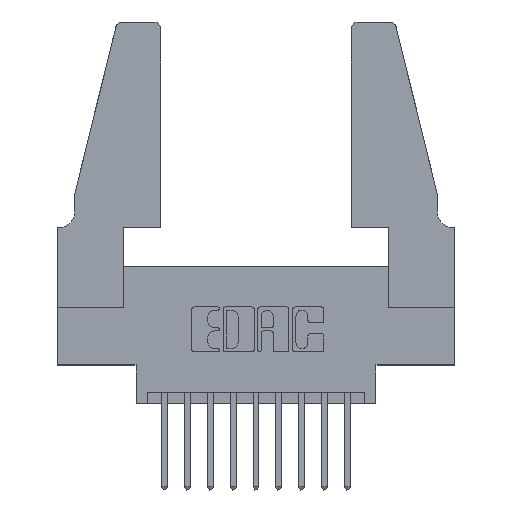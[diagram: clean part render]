
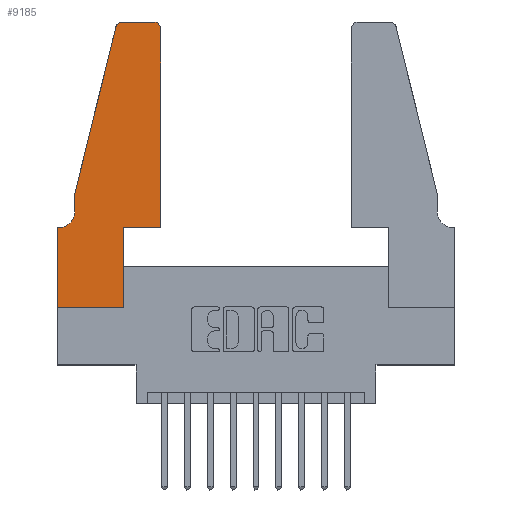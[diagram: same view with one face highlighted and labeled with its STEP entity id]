
A CAD part, top view. The second image highlights one B-rep face of the part: STEP entity #9185.
In plain terms, the highlighted planar face has unit normal (0, 0, 1).
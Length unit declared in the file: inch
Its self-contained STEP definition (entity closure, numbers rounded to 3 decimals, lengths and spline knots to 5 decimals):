
#111 = ORIENTED_EDGE ( 'NONE', *, *, #8602, .T. ) ;
#205 = FACE_OUTER_BOUND ( 'NONE', #3794, .T. ) ;
#253 = AXIS2_PLACEMENT_3D ( 'NONE', #5200, #1895, #12442 ) ;
#400 = EDGE_CURVE ( 'NONE', #8522, #9826, #4675, .T. ) ;
#411 = ORIENTED_EDGE ( 'NONE', *, *, #6340, .T. ) ;
#1037 = AXIS2_PLACEMENT_3D ( 'NONE', #12766, #9721, #3283 ) ;
#1057 = CARTESIAN_POINT ( 'NONE',  ( 0.284, 1.22, 0.37 ) ) ;
#1228 = CARTESIAN_POINT ( 'NONE',  ( 0., 0.35, 0.37 ) ) ;
#1343 = EDGE_CURVE ( 'NONE', #1656, #9816, #12976, .T. ) ;
#1396 = CARTESIAN_POINT ( 'NONE',  ( 0.2865, 0., 0.37 ) ) ;
#1656 = VERTEX_POINT ( 'NONE', #8082 ) ;
#1895 = DIRECTION ( 'NONE',  ( 0., 0., -1. ) ) ;
#2164 = ORIENTED_EDGE ( 'NONE', *, *, #400, .T. ) ;
#2370 = DIRECTION ( 'NONE',  ( -1., 0., 0. ) ) ;
#2409 = CARTESIAN_POINT ( 'NONE',  ( 0.4205, 1.25, 0.37 ) ) ;
#2418 = LINE ( 'NONE', #12150, #4247 ) ;
#2682 = CARTESIAN_POINT ( 'NONE',  ( 0.4505, 0.35, 0.37 ) ) ;
#2953 = CIRCLE ( 'NONE', #13236, 0.03 ) ;
#3154 = VERTEX_POINT ( 'NONE', #13482 ) ;
#3175 = CARTESIAN_POINT ( 'NONE',  ( 0.0755, 0.35, 0.37 ) ) ;
#3195 = LINE ( 'NONE', #11747, #11342 ) ;
#3283 = DIRECTION ( 'NONE',  ( 1., 0., 0. ) ) ;
#3365 = DIRECTION ( 'NONE',  ( 1., 0., 0. ) ) ;
#3552 = DIRECTION ( 'NONE',  ( 0., 0., 1. ) ) ;
#3661 = CARTESIAN_POINT ( 'NONE',  ( 0.4505, 1.22, 0.37 ) ) ;
#3710 = EDGE_CURVE ( 'NONE', #9374, #10309, #12224, .T. ) ;
#3794 = EDGE_LOOP ( 'NONE', ( #12296, #4757, #111, #2164, #6832, #6140, #9822, #10789, #10201, #5926, #411, #8245 ) ) ;
#4059 = DIRECTION ( 'NONE',  ( 0., 0., 1. ) ) ;
#4098 = CARTESIAN_POINT ( 'NONE',  ( 0.2865, 0.35, 0.37 ) ) ;
#4234 = DIRECTION ( 'NONE',  ( 0., 1., 0. ) ) ;
#4247 = VECTOR ( 'NONE', #11292, 39.37008 ) ;
#4675 = LINE ( 'NONE', #10441, #12673 ) ;
#4757 = ORIENTED_EDGE ( 'NONE', *, *, #11377, .T. ) ;
#4769 = CARTESIAN_POINT ( 'NONE',  ( 0., 0., 0.37 ) ) ;
#5063 = CARTESIAN_POINT ( 'NONE',  ( 0.284, 1.25, 0.37 ) ) ;
#5200 = CARTESIAN_POINT ( 'NONE',  ( 0.0055, 0.42, 0.37 ) ) ;
#5499 = VERTEX_POINT ( 'NONE', #10405 ) ;
#5926 = ORIENTED_EDGE ( 'NONE', *, *, #8165, .T. ) ;
#6053 = VECTOR ( 'NONE', #13142, 39.37008 ) ;
#6140 = ORIENTED_EDGE ( 'NONE', *, *, #1343, .T. ) ;
#6340 = EDGE_CURVE ( 'NONE', #3154, #7685, #3195, .T. ) ;
#6615 = AXIS2_PLACEMENT_3D ( 'NONE', #1057, #4059, #13797 ) ;
#6682 = LINE ( 'NONE', #12653, #11635 ) ;
#6832 = ORIENTED_EDGE ( 'NONE', *, *, #10294, .T. ) ;
#6933 = VERTEX_POINT ( 'NONE', #1396 ) ;
#7669 = CARTESIAN_POINT ( 'NONE',  ( 0.0755, 0.5, 0.37 ) ) ;
#7682 = CIRCLE ( 'NONE', #6615, 0.03 ) ;
#7685 = VERTEX_POINT ( 'NONE', #3661 ) ;
#7758 = DIRECTION ( 'NONE',  ( 1., 0., 0. ) ) ;
#7857 = CARTESIAN_POINT ( 'NONE',  ( 0.0755, 0.42, 0.37 ) ) ;
#8082 = CARTESIAN_POINT ( 'NONE',  ( 0.0055, 0.35, 0.37 ) ) ;
#8103 = VERTEX_POINT ( 'NONE', #13768 ) ;
#8165 = EDGE_CURVE ( 'NONE', #8103, #3154, #10397, .T. ) ;
#8245 = ORIENTED_EDGE ( 'NONE', *, *, #13560, .T. ) ;
#8505 = DIRECTION ( 'NONE',  ( 0., 1., 0. ) ) ;
#8522 = VERTEX_POINT ( 'NONE', #7669 ) ;
#8602 = EDGE_CURVE ( 'NONE', #5499, #8522, #2418, .T. ) ;
#8917 = EDGE_CURVE ( 'NONE', #6933, #8103, #9869, .T. ) ;
#9096 = CARTESIAN_POINT ( 'NONE',  ( 0., 0., 0.37 ) ) ;
#9185 = ADVANCED_FACE ( 'NONE', ( #205 ), #11766, .T. ) ;
#9374 = VERTEX_POINT ( 'NONE', #2409 ) ;
#9403 = VECTOR ( 'NONE', #2370, 39.37008 ) ;
#9515 = DIRECTION ( 'NONE',  ( 0., -1., 0. ) ) ;
#9562 = VECTOR ( 'NONE', #3365, 39.37008 ) ;
#9721 = DIRECTION ( 'NONE',  ( 0., 0., 1. ) ) ;
#9816 = VERTEX_POINT ( 'NONE', #1228 ) ;
#9822 = ORIENTED_EDGE ( 'NONE', *, *, #11852, .T. ) ;
#9826 = VERTEX_POINT ( 'NONE', #7857 ) ;
#9869 = LINE ( 'NONE', #4098, #13055 ) ;
#9917 = CARTESIAN_POINT ( 'NONE',  ( 0.4205, 1.22, 0.37 ) ) ;
#9920 = VERTEX_POINT ( 'NONE', #9096 ) ;
#10124 = CARTESIAN_POINT ( 'NONE',  ( 0.2605, 1.25, 0.37 ) ) ;
#10138 = VECTOR ( 'NONE', #11670, 39.37008 ) ;
#10201 = ORIENTED_EDGE ( 'NONE', *, *, #8917, .T. ) ;
#10294 = EDGE_CURVE ( 'NONE', #9826, #1656, #10993, .T. ) ;
#10309 = VERTEX_POINT ( 'NONE', #5063 ) ;
#10397 = LINE ( 'NONE', #2682, #9562 ) ;
#10405 = CARTESIAN_POINT ( 'NONE',  ( 0.25487, 1.22718, 0.37 ) ) ;
#10441 = CARTESIAN_POINT ( 'NONE',  ( 0.0755, 0.5, 0.37 ) ) ;
#10476 = EDGE_CURVE ( 'NONE', #9920, #6933, #13353, .T. ) ;
#10789 = ORIENTED_EDGE ( 'NONE', *, *, #10476, .T. ) ;
#10993 = CIRCLE ( 'NONE', #253, 0.07 ) ;
#11292 = DIRECTION ( 'NONE',  ( -0.239, -0.971, 0. ) ) ;
#11342 = VECTOR ( 'NONE', #4234, 39.37008 ) ;
#11377 = EDGE_CURVE ( 'NONE', #10309, #5499, #7682, .T. ) ;
#11635 = VECTOR ( 'NONE', #9515, 39.37008 ) ;
#11670 = DIRECTION ( 'NONE',  ( -1., 0., 0. ) ) ;
#11747 = CARTESIAN_POINT ( 'NONE',  ( 0.4505, 0.35, 0.37 ) ) ;
#11766 = PLANE ( 'NONE',  #1037 ) ;
#11852 = EDGE_CURVE ( 'NONE', #9816, #9920, #6682, .T. ) ;
#12150 = CARTESIAN_POINT ( 'NONE',  ( 0.0755, 0.5, 0.37 ) ) ;
#12224 = LINE ( 'NONE', #10124, #9403 ) ;
#12296 = ORIENTED_EDGE ( 'NONE', *, *, #3710, .T. ) ;
#12442 = DIRECTION ( 'NONE',  ( -1., 0., 0. ) ) ;
#12536 = DIRECTION ( 'NONE',  ( 0., -1., 0. ) ) ;
#12653 = CARTESIAN_POINT ( 'NONE',  ( 0., 0., 0.37 ) ) ;
#12673 = VECTOR ( 'NONE', #12536, 39.37008 ) ;
#12766 = CARTESIAN_POINT ( 'NONE',  ( 0., 0.35, 0.37 ) ) ;
#12976 = LINE ( 'NONE', #3175, #10138 ) ;
#13055 = VECTOR ( 'NONE', #8505, 39.37008 ) ;
#13142 = DIRECTION ( 'NONE',  ( 1., 0., 0. ) ) ;
#13236 = AXIS2_PLACEMENT_3D ( 'NONE', #9917, #3552, #7758 ) ;
#13353 = LINE ( 'NONE', #4769, #6053 ) ;
#13482 = CARTESIAN_POINT ( 'NONE',  ( 0.4505, 0.35, 0.37 ) ) ;
#13560 = EDGE_CURVE ( 'NONE', #7685, #9374, #2953, .T. ) ;
#13768 = CARTESIAN_POINT ( 'NONE',  ( 0.2865, 0.35, 0.37 ) ) ;
#13797 = DIRECTION ( 'NONE',  ( 1., 0., 0. ) ) ;
